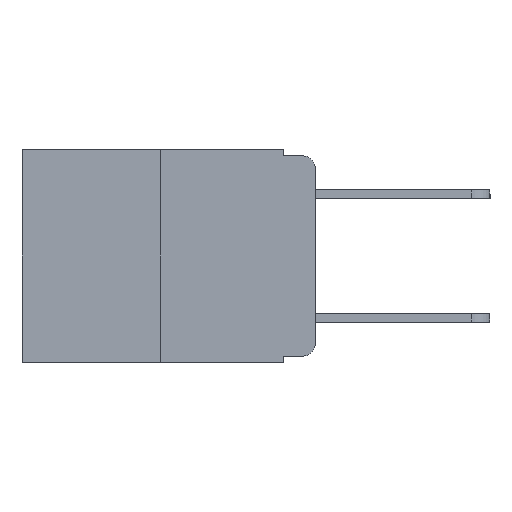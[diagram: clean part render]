
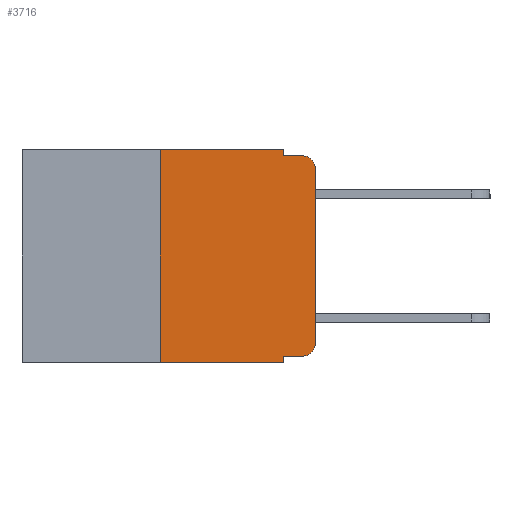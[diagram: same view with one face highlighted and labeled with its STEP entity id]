
A CAD part, left-side view. The second image highlights one B-rep face of the part: STEP entity #3716.
In plain terms, the highlighted planar face has unit normal (-1, 0, 0).
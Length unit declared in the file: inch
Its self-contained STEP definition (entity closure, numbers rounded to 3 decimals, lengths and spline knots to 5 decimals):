
#469 = FACE_OUTER_BOUND ( 'NONE', #11669, .T. ) ;
#622 = CARTESIAN_POINT ( 'NONE',  ( 0., 0.25, -0.343 ) ) ;
#998 = ORIENTED_EDGE ( 'NONE', *, *, #2856, .T. ) ;
#1040 = DIRECTION ( 'NONE',  ( 0., -1., 0. ) ) ;
#1747 = ORIENTED_EDGE ( 'NONE', *, *, #22234, .F. ) ;
#1854 = DIRECTION ( 'NONE',  ( 0., 0., -1. ) ) ;
#1911 = VECTOR ( 'NONE', #19456, 39.37008 ) ;
#2502 = CARTESIAN_POINT ( 'NONE',  ( 0., 0.051, 0. ) ) ;
#2856 = EDGE_CURVE ( 'NONE', #16781, #16391, #19352, .T. ) ;
#3122 = CARTESIAN_POINT ( 'NONE',  ( 0., 0.051, -0.01 ) ) ;
#3602 = VERTEX_POINT ( 'NONE', #11724 ) ;
#3716 = ADVANCED_FACE ( 'NONE', ( #469 ), #8245, .F. ) ;
#4527 = VERTEX_POINT ( 'NONE', #24287 ) ;
#4593 = CIRCLE ( 'NONE', #23602, 0.02 ) ;
#4915 = EDGE_CURVE ( 'NONE', #12059, #21851, #16946, .T. ) ;
#5242 = VECTOR ( 'NONE', #7865, 39.37008 ) ;
#5932 = DIRECTION ( 'NONE',  ( 0., 0., -1. ) ) ;
#6313 = CARTESIAN_POINT ( 'NONE',  ( 0., 0.473, 0. ) ) ;
#6402 = LINE ( 'NONE', #7555, #15914 ) ;
#6882 = LINE ( 'NONE', #2502, #1911 ) ;
#7347 = ORIENTED_EDGE ( 'NONE', *, *, #23273, .T. ) ;
#7555 = CARTESIAN_POINT ( 'NONE',  ( 0., 0.473, 0. ) ) ;
#7559 = ORIENTED_EDGE ( 'NONE', *, *, #11810, .T. ) ;
#7865 = DIRECTION ( 'NONE',  ( 0., 0., 1. ) ) ;
#8020 = ORIENTED_EDGE ( 'NONE', *, *, #4915, .T. ) ;
#8038 = AXIS2_PLACEMENT_3D ( 'NONE', #6313, #21394, #10157 ) ;
#8072 = DIRECTION ( 'NONE',  ( 0., 0., 1. ) ) ;
#8245 = PLANE ( 'NONE',  #8038 ) ;
#8366 = EDGE_CURVE ( 'NONE', #17733, #17567, #22086, .T. ) ;
#10157 = DIRECTION ( 'NONE',  ( 0., 0., -1. ) ) ;
#10464 = EDGE_CURVE ( 'NONE', #23891, #21897, #6402, .T. ) ;
#10523 = VECTOR ( 'NONE', #22731, 39.37008 ) ;
#10659 = CARTESIAN_POINT ( 'NONE',  ( 0., 0.02, -0.01 ) ) ;
#10983 = CARTESIAN_POINT ( 'NONE',  ( 0., 0.02, -0.313 ) ) ;
#11669 = EDGE_LOOP ( 'NONE', ( #7559, #7347, #12767, #22070, #17220, #1747, #998, #15929, #8020, #19587 ) ) ;
#11724 = CARTESIAN_POINT ( 'NONE',  ( 0., 0., -0.03 ) ) ;
#11810 = EDGE_CURVE ( 'NONE', #4527, #3602, #15347, .T. ) ;
#12013 = LINE ( 'NONE', #21213, #21959 ) ;
#12059 = VERTEX_POINT ( 'NONE', #18158 ) ;
#12151 = VECTOR ( 'NONE', #16341, 39.37008 ) ;
#12767 = ORIENTED_EDGE ( 'NONE', *, *, #8366, .F. ) ;
#12894 = DIRECTION ( 'NONE',  ( 0., 0., -1. ) ) ;
#13172 = DIRECTION ( 'NONE',  ( -1., 0., 0. ) ) ;
#13798 = AXIS2_PLACEMENT_3D ( 'NONE', #14316, #13172, #1854 ) ;
#14245 = CARTESIAN_POINT ( 'NONE',  ( 0., 0.051, -0.333 ) ) ;
#14316 = CARTESIAN_POINT ( 'NONE',  ( 0., 0.02, -0.03 ) ) ;
#14582 = CARTESIAN_POINT ( 'NONE',  ( 0., 0.051, -0.343 ) ) ;
#14927 = EDGE_CURVE ( 'NONE', #12059, #16391, #6882, .T. ) ;
#15315 = LINE ( 'NONE', #19186, #19711 ) ;
#15347 = LINE ( 'NONE', #19237, #5242 ) ;
#15357 = CARTESIAN_POINT ( 'NONE',  ( 0., 0.25, 0. ) ) ;
#15914 = VECTOR ( 'NONE', #20722, 39.37008 ) ;
#15929 = ORIENTED_EDGE ( 'NONE', *, *, #14927, .F. ) ;
#16341 = DIRECTION ( 'NONE',  ( 0., -1., 0. ) ) ;
#16391 = VERTEX_POINT ( 'NONE', #14582 ) ;
#16781 = VERTEX_POINT ( 'NONE', #622 ) ;
#16946 = LINE ( 'NONE', #14245, #21313 ) ;
#17220 = ORIENTED_EDGE ( 'NONE', *, *, #10464, .F. ) ;
#17567 = VERTEX_POINT ( 'NONE', #10659 ) ;
#17733 = VERTEX_POINT ( 'NONE', #20426 ) ;
#18158 = CARTESIAN_POINT ( 'NONE',  ( 0., 0.051, -0.333 ) ) ;
#19186 = CARTESIAN_POINT ( 'NONE',  ( 0., 0.051, 0. ) ) ;
#19237 = CARTESIAN_POINT ( 'NONE',  ( 0., 0., 0. ) ) ;
#19352 = LINE ( 'NONE', #20857, #10523 ) ;
#19456 = DIRECTION ( 'NONE',  ( 0., 0., -1. ) ) ;
#19587 = ORIENTED_EDGE ( 'NONE', *, *, #21899, .T. ) ;
#19711 = VECTOR ( 'NONE', #5932, 39.37008 ) ;
#20357 = EDGE_CURVE ( 'NONE', #21897, #17733, #15315, .T. ) ;
#20426 = CARTESIAN_POINT ( 'NONE',  ( 0., 0.051, -0.01 ) ) ;
#20722 = DIRECTION ( 'NONE',  ( 0., -1., 0. ) ) ;
#20857 = CARTESIAN_POINT ( 'NONE',  ( 0., 0.473, -0.343 ) ) ;
#21213 = CARTESIAN_POINT ( 'NONE',  ( 0., 0.25, 0. ) ) ;
#21313 = VECTOR ( 'NONE', #1040, 39.37008 ) ;
#21394 = DIRECTION ( 'NONE',  ( 1., 0., 0. ) ) ;
#21851 = VERTEX_POINT ( 'NONE', #23906 ) ;
#21897 = VERTEX_POINT ( 'NONE', #22109 ) ;
#21899 = EDGE_CURVE ( 'NONE', #21851, #4527, #4593, .T. ) ;
#21959 = VECTOR ( 'NONE', #8072, 39.37008 ) ;
#22070 = ORIENTED_EDGE ( 'NONE', *, *, #20357, .F. ) ;
#22086 = LINE ( 'NONE', #3122, #12151 ) ;
#22109 = CARTESIAN_POINT ( 'NONE',  ( 0., 0.051, 0. ) ) ;
#22234 = EDGE_CURVE ( 'NONE', #16781, #23891, #12013, .T. ) ;
#22731 = DIRECTION ( 'NONE',  ( 0., -1., 0. ) ) ;
#23273 = EDGE_CURVE ( 'NONE', #3602, #17567, #23361, .T. ) ;
#23361 = CIRCLE ( 'NONE', #13798, 0.02 ) ;
#23602 = AXIS2_PLACEMENT_3D ( 'NONE', #10983, #24067, #12894 ) ;
#23891 = VERTEX_POINT ( 'NONE', #15357 ) ;
#23906 = CARTESIAN_POINT ( 'NONE',  ( 0., 0.02, -0.333 ) ) ;
#24067 = DIRECTION ( 'NONE',  ( -1., 0., 0. ) ) ;
#24287 = CARTESIAN_POINT ( 'NONE',  ( 0., 0., -0.313 ) ) ;
